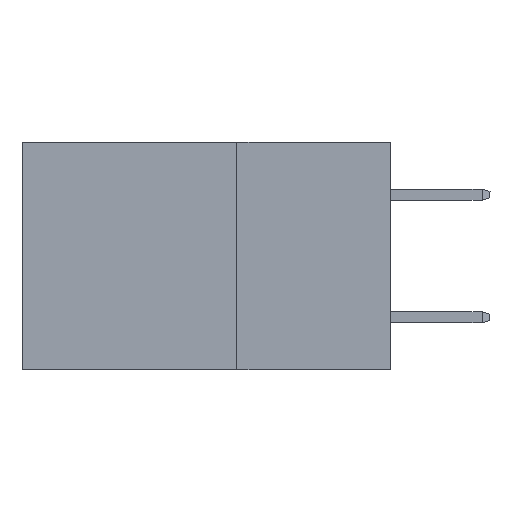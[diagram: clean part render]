
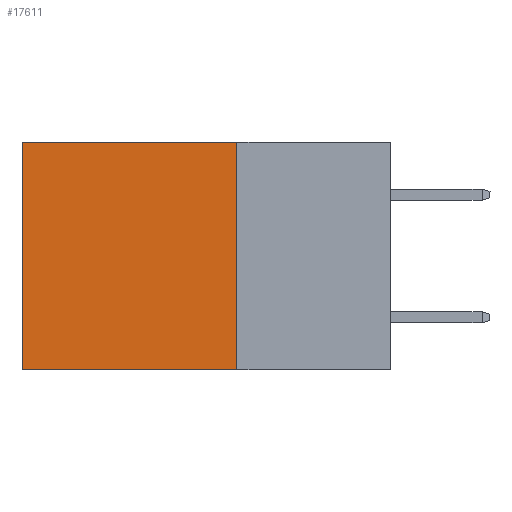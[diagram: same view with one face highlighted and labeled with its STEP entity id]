
A CAD part, left-side view. The second image highlights one B-rep face of the part: STEP entity #17611.
In plain terms, the highlighted planar face has unit normal (-1, 0, 0).
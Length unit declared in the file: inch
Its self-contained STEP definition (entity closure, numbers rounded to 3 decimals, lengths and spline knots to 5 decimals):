
#1732 = CARTESIAN_POINT ( 'NONE',  ( 0.2875, 0.25, 0. ) ) ;
#1837 = LINE ( 'NONE', #6688, #10084 ) ;
#3349 = DIRECTION ( 'NONE',  ( 0., 0., -1. ) ) ;
#4698 = VECTOR ( 'NONE', #10494, 39.37008 ) ;
#5104 = DIRECTION ( 'NONE',  ( 0., 0., -1. ) ) ;
#5770 = ORIENTED_EDGE ( 'NONE', *, *, #11914, .F. ) ;
#6096 = EDGE_CURVE ( 'NONE', #13293, #6791, #1837, .T. ) ;
#6688 = CARTESIAN_POINT ( 'NONE',  ( 0.2875, 0.25, 0. ) ) ;
#6791 = VERTEX_POINT ( 'NONE', #16563 ) ;
#7298 = VECTOR ( 'NONE', #13794, 39.37008 ) ;
#7807 = LINE ( 'NONE', #10500, #7298 ) ;
#8329 = DIRECTION ( 'NONE',  ( 0., 1., 0. ) ) ;
#8493 = EDGE_CURVE ( 'NONE', #6791, #20997, #18485, .T. ) ;
#10031 = ORIENTED_EDGE ( 'NONE', *, *, #13745, .F. ) ;
#10084 = VECTOR ( 'NONE', #8329, 39.37008 ) ;
#10494 = DIRECTION ( 'NONE',  ( 0., 0., -1. ) ) ;
#10500 = CARTESIAN_POINT ( 'NONE',  ( 0.2875, 0.25, -0.37 ) ) ;
#10847 = VERTEX_POINT ( 'NONE', #11263 ) ;
#11263 = CARTESIAN_POINT ( 'NONE',  ( 0.2875, 0.25, -0.37 ) ) ;
#11622 = PLANE ( 'NONE',  #19274 ) ;
#11914 = EDGE_CURVE ( 'NONE', #13293, #10847, #14030, .T. ) ;
#13240 = DIRECTION ( 'NONE',  ( 1., 0., 0. ) ) ;
#13293 = VERTEX_POINT ( 'NONE', #17531 ) ;
#13574 = ORIENTED_EDGE ( 'NONE', *, *, #8493, .T. ) ;
#13634 = ORIENTED_EDGE ( 'NONE', *, *, #6096, .T. ) ;
#13745 = EDGE_CURVE ( 'NONE', #10847, #20997, #7807, .T. ) ;
#13794 = DIRECTION ( 'NONE',  ( 0., 1., 0. ) ) ;
#13932 = FACE_OUTER_BOUND ( 'NONE', #15888, .T. ) ;
#14030 = LINE ( 'NONE', #18651, #4698 ) ;
#15888 = EDGE_LOOP ( 'NONE', ( #13574, #10031, #5770, #13634 ) ) ;
#16563 = CARTESIAN_POINT ( 'NONE',  ( 0.2875, 0.6, 0. ) ) ;
#16634 = CARTESIAN_POINT ( 'NONE',  ( 0.2875, 0.6, 0. ) ) ;
#17531 = CARTESIAN_POINT ( 'NONE',  ( 0.2875, 0.25, 0. ) ) ;
#17611 = ADVANCED_FACE ( 'NONE', ( #13932 ), #11622, .F. ) ;
#18485 = LINE ( 'NONE', #16634, #19010 ) ;
#18651 = CARTESIAN_POINT ( 'NONE',  ( 0.2875, 0.25, 0. ) ) ;
#19010 = VECTOR ( 'NONE', #5104, 39.37008 ) ;
#19274 = AXIS2_PLACEMENT_3D ( 'NONE', #1732, #13240, #3349 ) ;
#19307 = CARTESIAN_POINT ( 'NONE',  ( 0.2875, 0.6, -0.37 ) ) ;
#20997 = VERTEX_POINT ( 'NONE', #19307 ) ;
